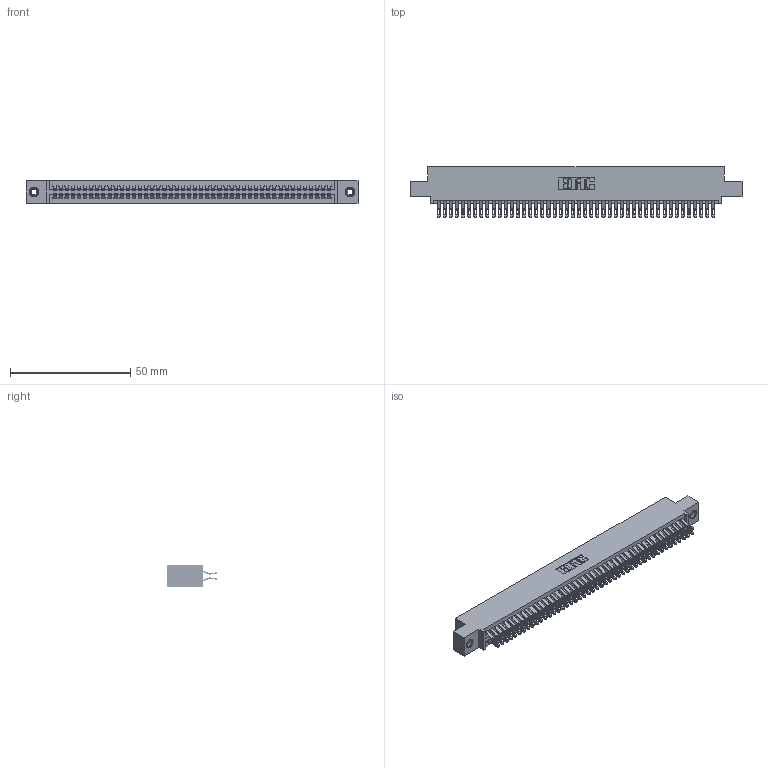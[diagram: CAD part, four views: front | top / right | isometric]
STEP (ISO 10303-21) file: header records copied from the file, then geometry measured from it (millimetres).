
FILE_DESCRIPTION (( 'STEP AP203' ), '1' );
FILE_NAME ('395-092-555-508.STEP', '2018-11-29T08:48:31', ( '' ), ( '' ), 'SwSTEP 2.0', 'SolidWorks 2016', '' );
FILE_SCHEMA (( 'CONFIG_CONTROL_DESIGN' ));
Length unit declared in the file: inch
Products named in the file (4): 345-292-001_555 Tail; 345-250-001_345-250-003-102; 395-092-555-508; 345 Part_0.110 Offset - 0.156 Dia-TI
Assembly tree (95 placements, depth 2):
  395-092-555-508
    345 Part_0.110 Offset - 0.156 Dia-TI
    345-292-001_555 Tail  x92
    345-250-001_345-250-003-102  x2
Bounding box: 138.05 x 21.13 x 9.4 mm (x, y, z)
Volume: 13634.3 mm3; surface area: 21265.7 mm2
Topology: 95 solids, 95 shells, 5342 faces, 16773 edges, 11174 vertices
Faces by surface type: plane 2968, cylinder 2358, cone 12, torus 4
Entity records: 37198 total; most frequent: CARTESIAN_POINT 6249, ORIENTED_EDGE 6146, DIRECTION 5499, EDGE_CURVE 3073, LINE 2717, VECTOR 2717, VERTEX_POINT 2044, AXIS2_PLACEMENT_3D 1391
